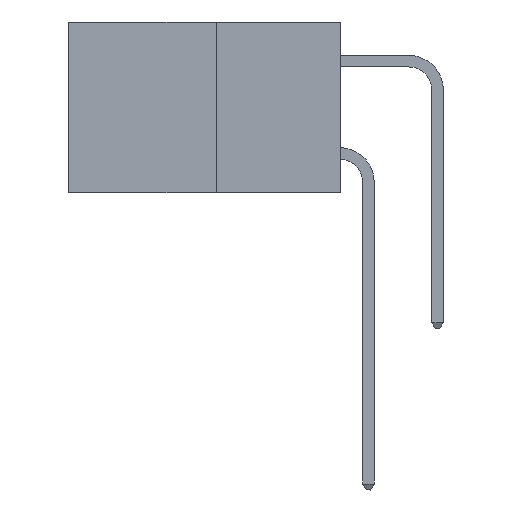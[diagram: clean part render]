
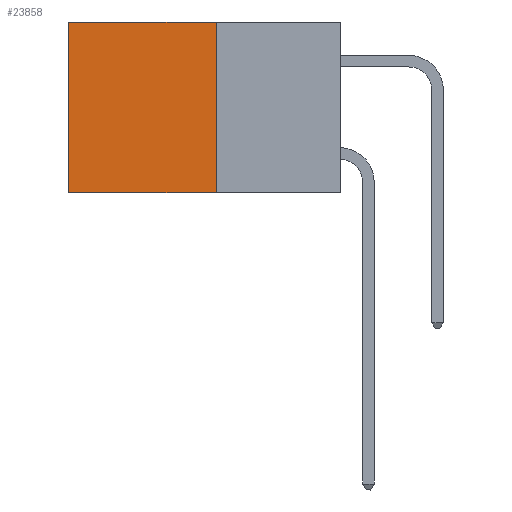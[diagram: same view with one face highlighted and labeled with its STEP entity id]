
A CAD part, left-side view. The second image highlights one B-rep face of the part: STEP entity #23858.
In plain terms, the highlighted planar face has unit normal (-1, 0, 0).
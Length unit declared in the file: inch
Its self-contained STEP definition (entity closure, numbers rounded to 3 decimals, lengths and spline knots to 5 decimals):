
#187 = CARTESIAN_POINT ( 'NONE',  ( 0.277, 0.59, 0. ) ) ;
#1038 = LINE ( 'NONE', #31777, #14121 ) ;
#2400 = CARTESIAN_POINT ( 'NONE',  ( 0.277, 0.27, -0.37 ) ) ;
#2561 = VERTEX_POINT ( 'NONE', #30746 ) ;
#2742 = DIRECTION ( 'NONE',  ( 0., 0., -1. ) ) ;
#3101 = CARTESIAN_POINT ( 'NONE',  ( 0.277, 0.59, -0.37 ) ) ;
#3666 = FACE_OUTER_BOUND ( 'NONE', #27259, .T. ) ;
#4065 = VECTOR ( 'NONE', #27083, 39.37008 ) ;
#4400 = AXIS2_PLACEMENT_3D ( 'NONE', #8374, #30250, #13978 ) ;
#5234 = DIRECTION ( 'NONE',  ( 0., 0., -1. ) ) ;
#5442 = PLANE ( 'NONE',  #4400 ) ;
#5931 = CARTESIAN_POINT ( 'NONE',  ( 0.277, 0.59, -0.37 ) ) ;
#7100 = ORIENTED_EDGE ( 'NONE', *, *, #7709, .T. ) ;
#7141 = VERTEX_POINT ( 'NONE', #5931 ) ;
#7344 = EDGE_CURVE ( 'NONE', #31113, #7141, #11021, .T. ) ;
#7709 = EDGE_CURVE ( 'NONE', #33225, #31113, #1038, .T. ) ;
#7837 = EDGE_CURVE ( 'NONE', #2561, #7141, #31491, .T. ) ;
#7838 = CARTESIAN_POINT ( 'NONE',  ( 0.277, 0.27, -0.37 ) ) ;
#8355 = ORIENTED_EDGE ( 'NONE', *, *, #35076, .F. ) ;
#8374 = CARTESIAN_POINT ( 'NONE',  ( 0.277, 0.27, -0.37 ) ) ;
#9142 = CARTESIAN_POINT ( 'NONE',  ( 0.277, 0.27, 0. ) ) ;
#11021 = LINE ( 'NONE', #3101, #24776 ) ;
#13978 = DIRECTION ( 'NONE',  ( 0., 0., -1. ) ) ;
#14121 = VECTOR ( 'NONE', #34245, 39.37008 ) ;
#23858 = ADVANCED_FACE ( 'NONE', ( #3666 ), #5442, .F. ) ;
#24776 = VECTOR ( 'NONE', #2742, 39.37008 ) ;
#27083 = DIRECTION ( 'NONE',  ( 0., 1., 0. ) ) ;
#27259 = EDGE_LOOP ( 'NONE', ( #34483, #32036, #8355, #7100 ) ) ;
#28175 = VECTOR ( 'NONE', #5234, 39.37008 ) ;
#30250 = DIRECTION ( 'NONE',  ( 1., 0., 0. ) ) ;
#30746 = CARTESIAN_POINT ( 'NONE',  ( 0.277, 0.27, -0.37 ) ) ;
#31113 = VERTEX_POINT ( 'NONE', #187 ) ;
#31491 = LINE ( 'NONE', #7838, #4065 ) ;
#31777 = CARTESIAN_POINT ( 'NONE',  ( 0.277, 0.27, 0. ) ) ;
#32036 = ORIENTED_EDGE ( 'NONE', *, *, #7837, .F. ) ;
#33225 = VERTEX_POINT ( 'NONE', #9142 ) ;
#34245 = DIRECTION ( 'NONE',  ( 0., 1., 0. ) ) ;
#34483 = ORIENTED_EDGE ( 'NONE', *, *, #7344, .T. ) ;
#35076 = EDGE_CURVE ( 'NONE', #33225, #2561, #35204, .T. ) ;
#35204 = LINE ( 'NONE', #2400, #28175 ) ;
